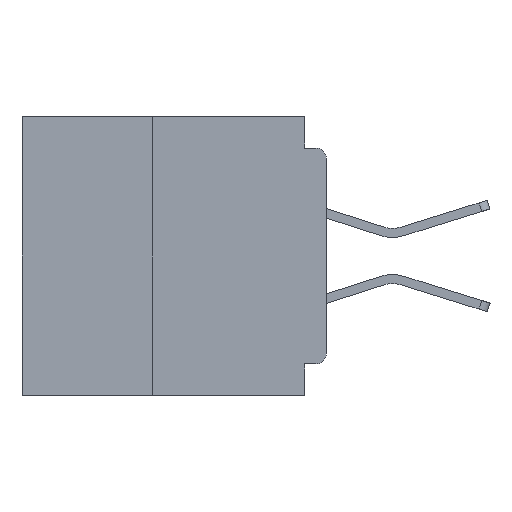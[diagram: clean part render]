
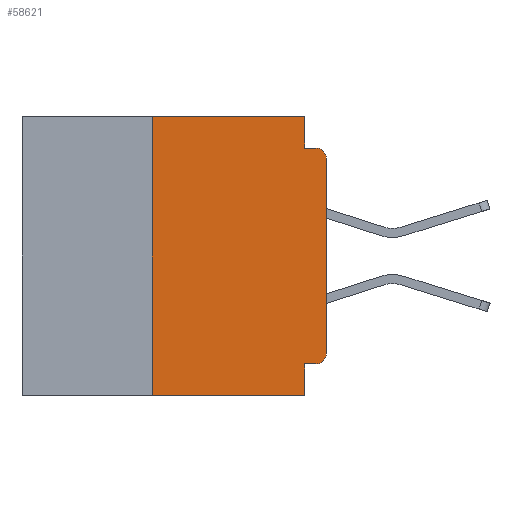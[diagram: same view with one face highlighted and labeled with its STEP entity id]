
A CAD part, left-side view. The second image highlights one B-rep face of the part: STEP entity #58621.
In plain terms, the highlighted planar face has unit normal (-1, 0, 0).
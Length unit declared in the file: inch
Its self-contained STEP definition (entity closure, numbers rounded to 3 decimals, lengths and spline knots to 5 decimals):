
#858 = ORIENTED_EDGE ( 'NONE', *, *, #10437, .F. ) ;
#7244 = VERTEX_POINT ( 'NONE', #53687 ) ;
#10437 = EDGE_CURVE ( 'NONE', #57183, #28332, #16402, .T. ) ;
#10968 = ORIENTED_EDGE ( 'NONE', *, *, #28048, .T. ) ;
#11667 = ORIENTED_EDGE ( 'NONE', *, *, #18983, .F. ) ;
#11886 = CARTESIAN_POINT ( 'NONE',  ( 0., 0.015, -0.045 ) ) ;
#12144 = EDGE_CURVE ( 'NONE', #29317, #57183, #55498, .T. ) ;
#12595 = DIRECTION ( 'NONE',  ( 0., 0., -1. ) ) ;
#13159 = DIRECTION ( 'NONE',  ( 0., 0., 1. ) ) ;
#13884 = DIRECTION ( 'NONE',  ( 0., -1., 0. ) ) ;
#15000 = VECTOR ( 'NONE', #44821, 39.37008 ) ;
#15612 = LINE ( 'NONE', #51496, #50923 ) ;
#16402 = LINE ( 'NONE', #53135, #51681 ) ;
#16716 = ORIENTED_EDGE ( 'NONE', *, *, #44152, .T. ) ;
#17159 = EDGE_LOOP ( 'NONE', ( #42686, #31869, #11667, #858, #17430, #58431, #10968, #47731, #51988, #16716 ) ) ;
#17430 = ORIENTED_EDGE ( 'NONE', *, *, #12144, .F. ) ;
#17542 = VERTEX_POINT ( 'NONE', #49533 ) ;
#17963 = VERTEX_POINT ( 'NONE', #32987 ) ;
#18983 = EDGE_CURVE ( 'NONE', #28332, #35576, #34197, .T. ) ;
#19861 = VERTEX_POINT ( 'NONE', #38448 ) ;
#20162 = CARTESIAN_POINT ( 'NONE',  ( 0., 0.031, -0.045 ) ) ;
#21590 = CARTESIAN_POINT ( 'NONE',  ( 0., 0., -0.355 ) ) ;
#22690 = CARTESIAN_POINT ( 'NONE',  ( 0., 0.25, 0. ) ) ;
#22976 = DIRECTION ( 'NONE',  ( 0., -1., 0. ) ) ;
#23448 = DIRECTION ( 'NONE',  ( -1., 0., 0. ) ) ;
#25590 = DIRECTION ( 'NONE',  ( 0., 0., -1. ) ) ;
#26150 = DIRECTION ( 'NONE',  ( 0., 0., 1. ) ) ;
#27031 = CARTESIAN_POINT ( 'NONE',  ( 0., 0.031, 0. ) ) ;
#27177 = EDGE_CURVE ( 'NONE', #19861, #29317, #52465, .T. ) ;
#27321 = LINE ( 'NONE', #21590, #15000 ) ;
#27434 = DIRECTION ( 'NONE',  ( -1., 0., 0. ) ) ;
#27668 = LINE ( 'NONE', #45446, #52081 ) ;
#27812 = CARTESIAN_POINT ( 'NONE',  ( 0., 0.015, -0.355 ) ) ;
#28022 = CARTESIAN_POINT ( 'NONE',  ( 0., 0.437, 0. ) ) ;
#28048 = EDGE_CURVE ( 'NONE', #19861, #43933, #29388, .T. ) ;
#28332 = VERTEX_POINT ( 'NONE', #20162 ) ;
#28749 = VERTEX_POINT ( 'NONE', #27812 ) ;
#29317 = VERTEX_POINT ( 'NONE', #22690 ) ;
#29388 = LINE ( 'NONE', #59595, #40235 ) ;
#30096 = EDGE_CURVE ( 'NONE', #28749, #17963, #27321, .T. ) ;
#31112 = VECTOR ( 'NONE', #13884, 39.37008 ) ;
#31869 = ORIENTED_EDGE ( 'NONE', *, *, #33357, .T. ) ;
#32142 = DIRECTION ( 'NONE',  ( 0., -1., 0. ) ) ;
#32868 = AXIS2_PLACEMENT_3D ( 'NONE', #35596, #40271, #12595 ) ;
#32987 = CARTESIAN_POINT ( 'NONE',  ( 0., 0.031, -0.355 ) ) ;
#33357 = EDGE_CURVE ( 'NONE', #7244, #35576, #41351, .T. ) ;
#34197 = LINE ( 'NONE', #55147, #57149 ) ;
#34842 = AXIS2_PLACEMENT_3D ( 'NONE', #54935, #27434, #59527 ) ;
#35576 = VERTEX_POINT ( 'NONE', #11886 ) ;
#35596 = CARTESIAN_POINT ( 'NONE',  ( 0., 0.437, 0. ) ) ;
#36927 = AXIS2_PLACEMENT_3D ( 'NONE', #51025, #23448, #55601 ) ;
#38448 = CARTESIAN_POINT ( 'NONE',  ( 0., 0.25, -0.4 ) ) ;
#40235 = VECTOR ( 'NONE', #32142, 39.37008 ) ;
#40271 = DIRECTION ( 'NONE',  ( 1., 0., 0. ) ) ;
#41351 = CIRCLE ( 'NONE', #34842, 0.015 ) ;
#41797 = VECTOR ( 'NONE', #26150, 39.37008 ) ;
#42538 = DIRECTION ( 'NONE',  ( 0., 0., -1. ) ) ;
#42686 = ORIENTED_EDGE ( 'NONE', *, *, #44545, .T. ) ;
#43933 = VERTEX_POINT ( 'NONE', #47777 ) ;
#44152 = EDGE_CURVE ( 'NONE', #28749, #17542, #49307, .T. ) ;
#44545 = EDGE_CURVE ( 'NONE', #17542, #7244, #27668, .T. ) ;
#44821 = DIRECTION ( 'NONE',  ( 0., 1., 0. ) ) ;
#45446 = CARTESIAN_POINT ( 'NONE',  ( 0., 0., 0. ) ) ;
#47731 = ORIENTED_EDGE ( 'NONE', *, *, #57400, .F. ) ;
#47777 = CARTESIAN_POINT ( 'NONE',  ( 0., 0.031, -0.4 ) ) ;
#49095 = CARTESIAN_POINT ( 'NONE',  ( 0., 0.25, -0.4 ) ) ;
#49307 = CIRCLE ( 'NONE', #36927, 0.015 ) ;
#49533 = CARTESIAN_POINT ( 'NONE',  ( 0., 0., -0.34 ) ) ;
#50923 = VECTOR ( 'NONE', #42538, 39.37008 ) ;
#51025 = CARTESIAN_POINT ( 'NONE',  ( 0., 0.015, -0.34 ) ) ;
#51496 = CARTESIAN_POINT ( 'NONE',  ( 0., 0.031, -0.4 ) ) ;
#51681 = VECTOR ( 'NONE', #25590, 39.37008 ) ;
#51988 = ORIENTED_EDGE ( 'NONE', *, *, #30096, .F. ) ;
#52081 = VECTOR ( 'NONE', #13159, 39.37008 ) ;
#52465 = LINE ( 'NONE', #49095, #41797 ) ;
#53135 = CARTESIAN_POINT ( 'NONE',  ( 0., 0.031, 0. ) ) ;
#53687 = CARTESIAN_POINT ( 'NONE',  ( 0., 0., -0.06 ) ) ;
#53852 = PLANE ( 'NONE',  #32868 ) ;
#54935 = CARTESIAN_POINT ( 'NONE',  ( 0., 0.015, -0.06 ) ) ;
#55147 = CARTESIAN_POINT ( 'NONE',  ( 0., 0., -0.045 ) ) ;
#55498 = LINE ( 'NONE', #28022, #31112 ) ;
#55601 = DIRECTION ( 'NONE',  ( 0., 0., -1. ) ) ;
#56474 = FACE_OUTER_BOUND ( 'NONE', #17159, .T. ) ;
#57149 = VECTOR ( 'NONE', #22976, 39.37008 ) ;
#57183 = VERTEX_POINT ( 'NONE', #27031 ) ;
#57400 = EDGE_CURVE ( 'NONE', #17963, #43933, #15612, .T. ) ;
#58431 = ORIENTED_EDGE ( 'NONE', *, *, #27177, .F. ) ;
#58621 = ADVANCED_FACE ( 'NONE', ( #56474 ), #53852, .F. ) ;
#59527 = DIRECTION ( 'NONE',  ( 0., 0., -1. ) ) ;
#59595 = CARTESIAN_POINT ( 'NONE',  ( 0., 0.437, -0.4 ) ) ;
